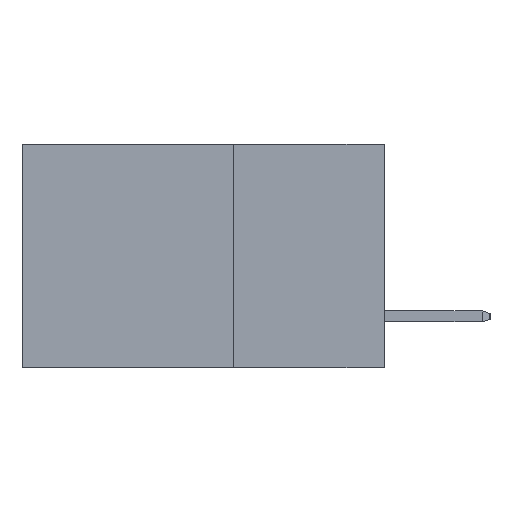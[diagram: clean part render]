
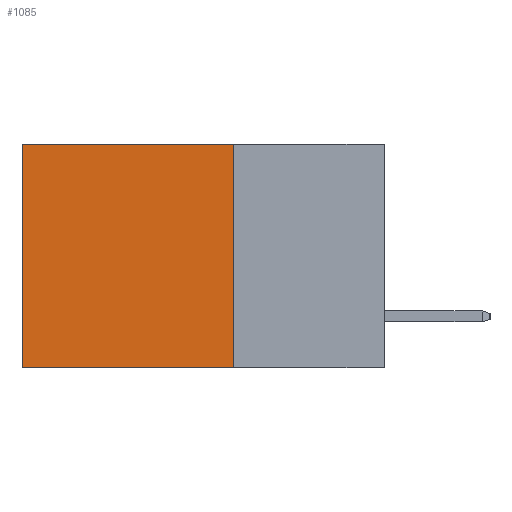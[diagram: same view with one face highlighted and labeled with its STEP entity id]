
A CAD part, left-side view. The second image highlights one B-rep face of the part: STEP entity #1085.
In plain terms, the highlighted planar face has unit normal (-1, 0, 0).
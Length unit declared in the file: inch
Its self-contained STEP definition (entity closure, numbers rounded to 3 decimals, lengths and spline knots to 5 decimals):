
#100 = ORIENTED_EDGE ( 'NONE', *, *, #16629, .T. ) ;
#116 = ORIENTED_EDGE ( 'NONE', *, *, #6655, .F. ) ;
#936 = DIRECTION ( 'NONE',  ( 0., 0., -1. ) ) ;
#1085 = ADVANCED_FACE ( 'NONE', ( #5561 ), #19471, .F. ) ;
#1246 = CARTESIAN_POINT ( 'NONE',  ( 0.298, 0.25, 0. ) ) ;
#1294 = DIRECTION ( 'NONE',  ( 1., 0., 0. ) ) ;
#3180 = DIRECTION ( 'NONE',  ( 0., 1., 0. ) ) ;
#3225 = VERTEX_POINT ( 'NONE', #1246 ) ;
#4261 = EDGE_CURVE ( 'NONE', #3225, #18234, #17147, .T. ) ;
#4794 = CARTESIAN_POINT ( 'NONE',  ( 0.298, 0.6, 0. ) ) ;
#5561 = FACE_OUTER_BOUND ( 'NONE', #22054, .T. ) ;
#6655 = EDGE_CURVE ( 'NONE', #18234, #19072, #7175, .T. ) ;
#6669 = DIRECTION ( 'NONE',  ( 0., 0., -1. ) ) ;
#7070 = LINE ( 'NONE', #11957, #7625 ) ;
#7175 = LINE ( 'NONE', #15379, #20134 ) ;
#7436 = CARTESIAN_POINT ( 'NONE',  ( 0.298, 0.6, 0. ) ) ;
#7490 = CARTESIAN_POINT ( 'NONE',  ( 0.298, 0.25, 0. ) ) ;
#7506 = DIRECTION ( 'NONE',  ( 0., 0., -1. ) ) ;
#7625 = VECTOR ( 'NONE', #3180, 39.37008 ) ;
#7791 = CARTESIAN_POINT ( 'NONE',  ( 0.298, 0.25, -0.37 ) ) ;
#7799 = EDGE_CURVE ( 'NONE', #17207, #19072, #13866, .T. ) ;
#9333 = VECTOR ( 'NONE', #7506, 39.37008 ) ;
#11957 = CARTESIAN_POINT ( 'NONE',  ( 0.298, 0.25, 0. ) ) ;
#12451 = CARTESIAN_POINT ( 'NONE',  ( 0.298, 0.6, -0.37 ) ) ;
#13866 = LINE ( 'NONE', #7436, #9333 ) ;
#14235 = ORIENTED_EDGE ( 'NONE', *, *, #4261, .F. ) ;
#14573 = DIRECTION ( 'NONE',  ( 0., 1., 0. ) ) ;
#15379 = CARTESIAN_POINT ( 'NONE',  ( 0.298, 0.25, -0.37 ) ) ;
#15497 = AXIS2_PLACEMENT_3D ( 'NONE', #21783, #1294, #6669 ) ;
#16629 = EDGE_CURVE ( 'NONE', #3225, #17207, #7070, .T. ) ;
#16762 = ORIENTED_EDGE ( 'NONE', *, *, #7799, .T. ) ;
#17147 = LINE ( 'NONE', #7490, #20976 ) ;
#17207 = VERTEX_POINT ( 'NONE', #4794 ) ;
#18234 = VERTEX_POINT ( 'NONE', #7791 ) ;
#19072 = VERTEX_POINT ( 'NONE', #12451 ) ;
#19471 = PLANE ( 'NONE',  #15497 ) ;
#20134 = VECTOR ( 'NONE', #14573, 39.37008 ) ;
#20976 = VECTOR ( 'NONE', #936, 39.37008 ) ;
#21783 = CARTESIAN_POINT ( 'NONE',  ( 0.298, 0.25, 0. ) ) ;
#22054 = EDGE_LOOP ( 'NONE', ( #16762, #116, #14235, #100 ) ) ;
